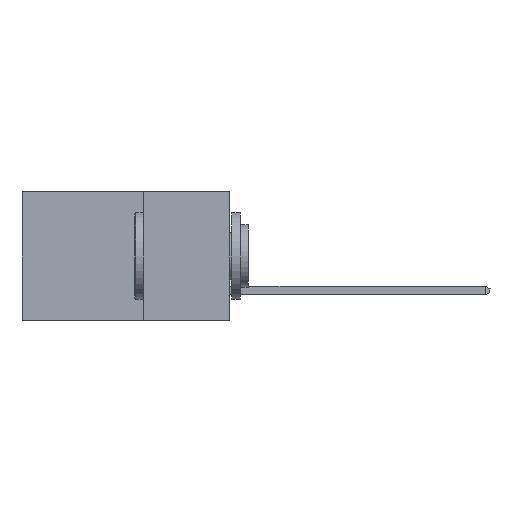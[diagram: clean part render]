
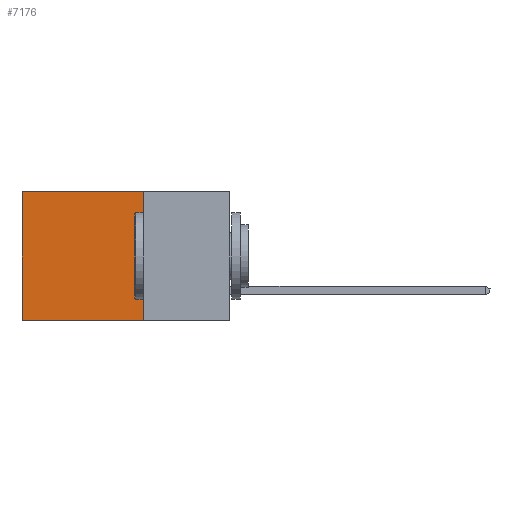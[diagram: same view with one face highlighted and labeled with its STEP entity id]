
A CAD part, left-side view. The second image highlights one B-rep face of the part: STEP entity #7176.
In plain terms, the highlighted planar face has unit normal (-1, 0, 0).
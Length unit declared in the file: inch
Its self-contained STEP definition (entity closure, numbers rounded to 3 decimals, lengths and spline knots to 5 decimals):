
#86 = DIRECTION ( 'NONE',  ( 0., 0., -1. ) ) ;
#389 = EDGE_CURVE ( 'NONE', #6626, #14048, #6184, .T. ) ;
#1886 = ORIENTED_EDGE ( 'NONE', *, *, #14209, .F. ) ;
#1948 = VERTEX_POINT ( 'NONE', #9981 ) ;
#2196 = ORIENTED_EDGE ( 'NONE', *, *, #389, .T. ) ;
#3325 = CARTESIAN_POINT ( 'NONE',  ( 0.2615, 0.25, -0.37 ) ) ;
#3573 = CARTESIAN_POINT ( 'NONE',  ( 0.2615, 0.25, 0. ) ) ;
#3785 = DIRECTION ( 'NONE',  ( 1., 0., 0. ) ) ;
#4032 = DIRECTION ( 'NONE',  ( 0., 0., -1. ) ) ;
#4695 = LINE ( 'NONE', #12847, #7078 ) ;
#5343 = EDGE_CURVE ( 'NONE', #6626, #13001, #14231, .T. ) ;
#6184 = LINE ( 'NONE', #18688, #20973 ) ;
#6626 = VERTEX_POINT ( 'NONE', #3573 ) ;
#7078 = VECTOR ( 'NONE', #8612, 39.37008 ) ;
#7176 = ADVANCED_FACE ( 'NONE', ( #20939 ), #13334, .F. ) ;
#8612 = DIRECTION ( 'NONE',  ( 0., 1., 0. ) ) ;
#9129 = CARTESIAN_POINT ( 'NONE',  ( 0.2615, 0.6, -0.37 ) ) ;
#9981 = CARTESIAN_POINT ( 'NONE',  ( 0.2615, 0.6, -0.37 ) ) ;
#10073 = CARTESIAN_POINT ( 'NONE',  ( 0.2615, 0.6, 0. ) ) ;
#10327 = ORIENTED_EDGE ( 'NONE', *, *, #15172, .T. ) ;
#10787 = EDGE_LOOP ( 'NONE', ( #10327, #1886, #18273, #2196 ) ) ;
#11192 = DIRECTION ( 'NONE',  ( 0., 1., 0. ) ) ;
#12847 = CARTESIAN_POINT ( 'NONE',  ( 0.2615, 0.25, -0.37 ) ) ;
#13001 = VERTEX_POINT ( 'NONE', #15604 ) ;
#13334 = PLANE ( 'NONE',  #21936 ) ;
#14048 = VERTEX_POINT ( 'NONE', #10073 ) ;
#14070 = VECTOR ( 'NONE', #86, 39.37008 ) ;
#14209 = EDGE_CURVE ( 'NONE', #13001, #1948, #4695, .T. ) ;
#14231 = LINE ( 'NONE', #3325, #14070 ) ;
#15172 = EDGE_CURVE ( 'NONE', #14048, #1948, #16841, .T. ) ;
#15604 = CARTESIAN_POINT ( 'NONE',  ( 0.2615, 0.25, -0.37 ) ) ;
#16841 = LINE ( 'NONE', #9129, #19242 ) ;
#18273 = ORIENTED_EDGE ( 'NONE', *, *, #5343, .F. ) ;
#18451 = DIRECTION ( 'NONE',  ( 0., 0., -1. ) ) ;
#18688 = CARTESIAN_POINT ( 'NONE',  ( 0.2615, 0.25, 0. ) ) ;
#19242 = VECTOR ( 'NONE', #18451, 39.37008 ) ;
#20580 = CARTESIAN_POINT ( 'NONE',  ( 0.2615, 0.25, -0.37 ) ) ;
#20939 = FACE_OUTER_BOUND ( 'NONE', #10787, .T. ) ;
#20973 = VECTOR ( 'NONE', #11192, 39.37008 ) ;
#21936 = AXIS2_PLACEMENT_3D ( 'NONE', #20580, #3785, #4032 ) ;
